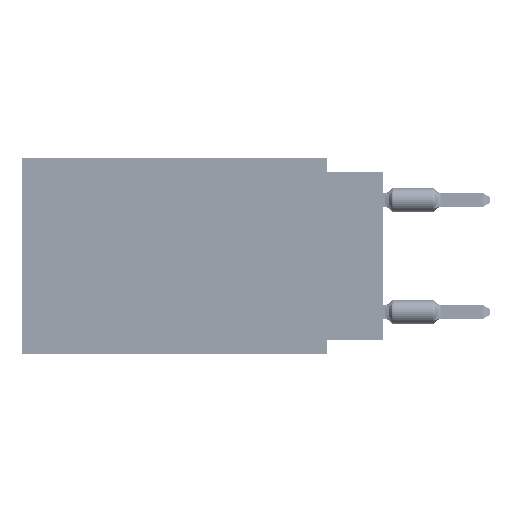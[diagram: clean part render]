
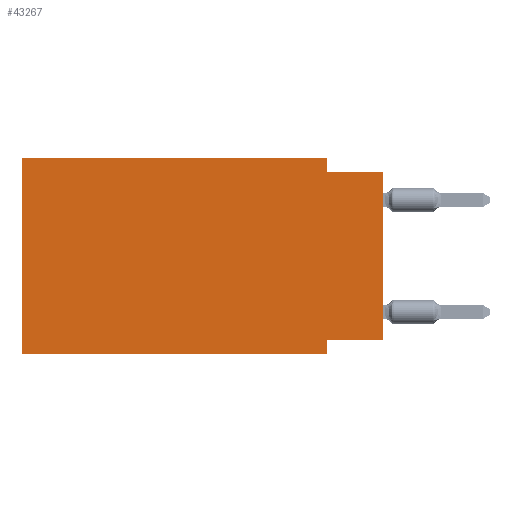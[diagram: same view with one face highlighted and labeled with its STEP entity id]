
A CAD part, left-side view. The second image highlights one B-rep face of the part: STEP entity #43267.
In plain terms, the highlighted planar face has unit normal (-1, 0, 0).
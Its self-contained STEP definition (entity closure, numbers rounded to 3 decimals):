
#535 = VERTEX_POINT ( 'NONE', #23402 ) ;
#2970 = ORIENTED_EDGE ( 'NONE', *, *, #37136, .F. ) ;
#6064 = CARTESIAN_POINT ( 'NONE',  ( 0., 16.383, -8.89 ) ) ;
#7427 = DIRECTION ( 'NONE',  ( 0., 1., 0. ) ) ;
#13041 = DIRECTION ( 'NONE',  ( 0., 0., 1. ) ) ;
#13147 = CARTESIAN_POINT ( 'NONE',  ( 0., 0., -8.255 ) ) ;
#15149 = LINE ( 'NONE', #43271, #30932 ) ;
#15520 = DIRECTION ( 'NONE',  ( 0., -1., 0. ) ) ;
#15553 = DIRECTION ( 'NONE',  ( 0., 0., -1. ) ) ;
#16347 = ORIENTED_EDGE ( 'NONE', *, *, #37035, .T. ) ;
#18548 = VERTEX_POINT ( 'NONE', #20835 ) ;
#19442 = DIRECTION ( 'NONE',  ( 0., -1., 0. ) ) ;
#19908 = LINE ( 'NONE', #48015, #74736 ) ;
#20835 = CARTESIAN_POINT ( 'NONE',  ( 0., 2.54, -8.89 ) ) ;
#22022 = LINE ( 'NONE', #34129, #47426 ) ;
#22359 = EDGE_CURVE ( 'NONE', #33708, #18548, #22022, .T. ) ;
#23402 = CARTESIAN_POINT ( 'NONE',  ( 0., 16.383, 0. ) ) ;
#23997 = AXIS2_PLACEMENT_3D ( 'NONE', #65852, #29449, #80115 ) ;
#24878 = VERTEX_POINT ( 'NONE', #61651 ) ;
#27600 = CARTESIAN_POINT ( 'NONE',  ( 0., 0., 0. ) ) ;
#29449 = DIRECTION ( 'NONE',  ( 1., 0., 0. ) ) ;
#30445 = EDGE_CURVE ( 'NONE', #535, #70226, #64385, .T. ) ;
#30932 = VECTOR ( 'NONE', #71391, 1000. ) ;
#30983 = ORIENTED_EDGE ( 'NONE', *, *, #71861, .T. ) ;
#33708 = VERTEX_POINT ( 'NONE', #37367 ) ;
#34129 = CARTESIAN_POINT ( 'NONE',  ( 0., 2.54, -8.89 ) ) ;
#37035 = EDGE_CURVE ( 'NONE', #56905, #18548, #39738, .T. ) ;
#37136 = EDGE_CURVE ( 'NONE', #70226, #58383, #19908, .T. ) ;
#37321 = VECTOR ( 'NONE', #15520, 1000. ) ;
#37367 = CARTESIAN_POINT ( 'NONE',  ( 0., 2.54, -8.255 ) ) ;
#37401 = VECTOR ( 'NONE', #7427, 1000. ) ;
#37739 = PLANE ( 'NONE',  #23997 ) ;
#39738 = LINE ( 'NONE', #6064, #86514 ) ;
#40378 = ORIENTED_EDGE ( 'NONE', *, *, #84460, .F. ) ;
#41063 = CARTESIAN_POINT ( 'NONE',  ( 0., 2.54, 0. ) ) ;
#41532 = ORIENTED_EDGE ( 'NONE', *, *, #22359, .F. ) ;
#43267 = ADVANCED_FACE ( 'NONE', ( #85210 ), #37739, .F. ) ;
#43271 = CARTESIAN_POINT ( 'NONE',  ( 0., 0., -0.635 ) ) ;
#44992 = CARTESIAN_POINT ( 'NONE',  ( 0., 2.54, -0.635 ) ) ;
#45269 = ORIENTED_EDGE ( 'NONE', *, *, #68303, .F. ) ;
#47426 = VECTOR ( 'NONE', #15553, 1000. ) ;
#48015 = CARTESIAN_POINT ( 'NONE',  ( 0., 2.54, 0. ) ) ;
#48062 = LINE ( 'NONE', #76177, #77197 ) ;
#49250 = EDGE_LOOP ( 'NONE', ( #30983, #40378, #2970, #55142, #88216, #16347, #41532, #45269 ) ) ;
#53377 = VECTOR ( 'NONE', #69537, 1000. ) ;
#55142 = ORIENTED_EDGE ( 'NONE', *, *, #30445, .F. ) ;
#56172 = LINE ( 'NONE', #27600, #53377 ) ;
#56905 = VERTEX_POINT ( 'NONE', #63012 ) ;
#57466 = CARTESIAN_POINT ( 'NONE',  ( 0., 16.383, 0. ) ) ;
#58383 = VERTEX_POINT ( 'NONE', #44992 ) ;
#61651 = CARTESIAN_POINT ( 'NONE',  ( 0., 0., -0.635 ) ) ;
#63012 = CARTESIAN_POINT ( 'NONE',  ( 0., 16.383, -8.89 ) ) ;
#63229 = EDGE_CURVE ( 'NONE', #56905, #535, #48062, .T. ) ;
#63677 = CARTESIAN_POINT ( 'NONE',  ( 0., 0., -8.255 ) ) ;
#64385 = LINE ( 'NONE', #57466, #37321 ) ;
#64594 = LINE ( 'NONE', #63677, #37401 ) ;
#65852 = CARTESIAN_POINT ( 'NONE',  ( 0., 16.383, 0. ) ) ;
#68303 = EDGE_CURVE ( 'NONE', #79687, #33708, #64594, .T. ) ;
#69537 = DIRECTION ( 'NONE',  ( 0., 0., 1. ) ) ;
#70226 = VERTEX_POINT ( 'NONE', #41063 ) ;
#71391 = DIRECTION ( 'NONE',  ( 0., -1., 0. ) ) ;
#71861 = EDGE_CURVE ( 'NONE', #79687, #24878, #56172, .T. ) ;
#74736 = VECTOR ( 'NONE', #76129, 1000. ) ;
#76129 = DIRECTION ( 'NONE',  ( 0., 0., -1. ) ) ;
#76177 = CARTESIAN_POINT ( 'NONE',  ( 0., 16.383, 0. ) ) ;
#77197 = VECTOR ( 'NONE', #13041, 1000. ) ;
#79687 = VERTEX_POINT ( 'NONE', #13147 ) ;
#80115 = DIRECTION ( 'NONE',  ( 0., 0., -1. ) ) ;
#84460 = EDGE_CURVE ( 'NONE', #58383, #24878, #15149, .T. ) ;
#85210 = FACE_OUTER_BOUND ( 'NONE', #49250, .T. ) ;
#86514 = VECTOR ( 'NONE', #19442, 1000. ) ;
#88216 = ORIENTED_EDGE ( 'NONE', *, *, #63229, .F. ) ;
